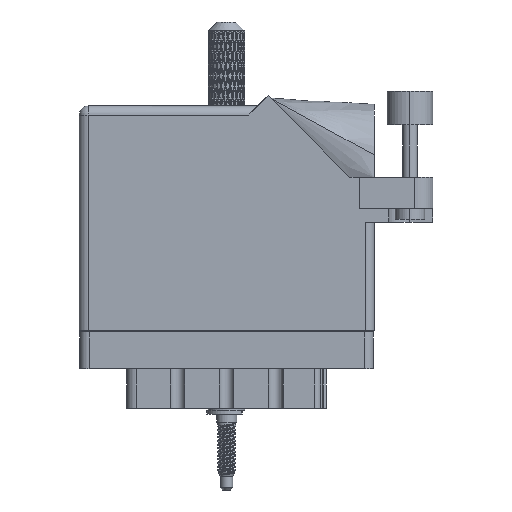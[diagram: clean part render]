
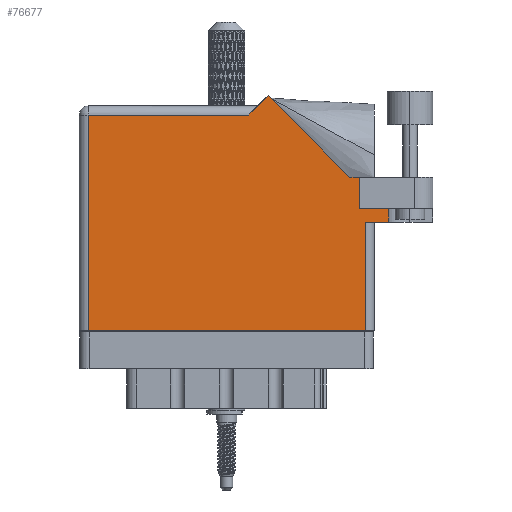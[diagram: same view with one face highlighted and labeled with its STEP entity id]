
A CAD part, front view. The second image highlights one B-rep face of the part: STEP entity #76677.
In plain terms, the highlighted face is planar.
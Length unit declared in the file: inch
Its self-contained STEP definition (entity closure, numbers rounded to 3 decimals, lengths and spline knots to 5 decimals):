
#57 = VECTOR ( 'NONE', #5268, 39.37008 ) ;
#938 = CARTESIAN_POINT ( 'NONE',  ( 0., 1.468, 0. ) ) ;
#1579 = LINE ( 'NONE', #55745, #51503 ) ;
#4344 = VECTOR ( 'NONE', #47164, 39.37008 ) ;
#4635 = DIRECTION ( 'NONE',  ( 1., 0., 0. ) ) ;
#5253 = VERTEX_POINT ( 'NONE', #78853 ) ;
#5268 = DIRECTION ( 'NONE',  ( -0.707, 0.707, 0. ) ) ;
#8035 = VERTEX_POINT ( 'NONE', #67696 ) ;
#8928 = VERTEX_POINT ( 'NONE', #51067 ) ;
#10046 = EDGE_CURVE ( 'NONE', #5253, #21552, #40392, .T. ) ;
#19671 = CARTESIAN_POINT ( 'NONE',  ( 1.948, 0.737, 0. ) ) ;
#21103 = DIRECTION ( 'NONE',  ( 1., 0., 0. ) ) ;
#21552 = VERTEX_POINT ( 'NONE', #83083 ) ;
#22017 = CARTESIAN_POINT ( 'NONE',  ( 1.84442, 1.044, 0. ) ) ;
#22342 = EDGE_CURVE ( 'NONE', #89152, #8035, #93505, .T. ) ;
#23425 = ORIENTED_EDGE ( 'NONE', *, *, #70591, .T. ) ;
#23950 = EDGE_CURVE ( 'NONE', #89152, #102067, #57091, .T. ) ;
#25335 = VERTEX_POINT ( 'NONE', #33425 ) ;
#25828 = VECTOR ( 'NONE', #78923, 39.37008 ) ;
#27591 = CARTESIAN_POINT ( 'NONE',  ( 0., 1.53, 0. ) ) ;
#28044 = VECTOR ( 'NONE', #87202, 39.37008 ) ;
#28593 = VECTOR ( 'NONE', #63120, 39.37008 ) ;
#28971 = CARTESIAN_POINT ( 'NONE',  ( 2.41, 1.044, 0. ) ) ;
#29723 = ORIENTED_EDGE ( 'NONE', *, *, #41947, .T. ) ;
#30612 = DIRECTION ( 'NONE',  ( 0., -1., 0. ) ) ;
#31033 = VECTOR ( 'NONE', #4635, 39.37008 ) ;
#32661 = EDGE_CURVE ( 'NONE', #8035, #25335, #1579, .T. ) ;
#32715 = ORIENTED_EDGE ( 'NONE', *, *, #77418, .T. ) ;
#33425 = CARTESIAN_POINT ( 'NONE',  ( 2.1115, 0.737, 0. ) ) ;
#34842 = VERTEX_POINT ( 'NONE', #71585 ) ;
#35898 = ORIENTED_EDGE ( 'NONE', *, *, #38329, .T. ) ;
#36081 = FACE_OUTER_BOUND ( 'NONE', #95447, .T. ) ;
#38329 = EDGE_CURVE ( 'NONE', #48681, #8928, #70773, .T. ) ;
#38809 = CARTESIAN_POINT ( 'NONE',  ( 1.948, 0.737, 0. ) ) ;
#40392 = LINE ( 'NONE', #938, #86519 ) ;
#41947 = EDGE_CURVE ( 'NONE', #82631, #25335, #71686, .T. ) ;
#42359 = LINE ( 'NONE', #66428, #62415 ) ;
#43043 = LINE ( 'NONE', #28971, #64299 ) ;
#43227 = CARTESIAN_POINT ( 'NONE',  ( 0.062, 0., 0. ) ) ;
#44780 = VERTEX_POINT ( 'NONE', #95991 ) ;
#47164 = DIRECTION ( 'NONE',  ( 0., 1., 0. ) ) ;
#47838 = ORIENTED_EDGE ( 'NONE', *, *, #75575, .T. ) ;
#48681 = VERTEX_POINT ( 'NONE', #43227 ) ;
#49773 = LINE ( 'NONE', #71113, #28593 ) ;
#50379 = CARTESIAN_POINT ( 'NONE',  ( 1.91, 1.044, 0. ) ) ;
#51067 = CARTESIAN_POINT ( 'NONE',  ( 1.948, 0., 0. ) ) ;
#51503 = VECTOR ( 'NONE', #30612, 39.37008 ) ;
#52007 = DIRECTION ( 'NONE',  ( 0., 0., -1. ) ) ;
#52464 = ORIENTED_EDGE ( 'NONE', *, *, #23950, .T. ) ;
#53269 = EDGE_CURVE ( 'NONE', #21552, #48681, #42359, .T. ) ;
#55745 = CARTESIAN_POINT ( 'NONE',  ( 2.1115, 1.16177, 0. ) ) ;
#56846 = CARTESIAN_POINT ( 'NONE',  ( 1.91, 0.831, 0. ) ) ;
#57091 = LINE ( 'NONE', #86573, #25828 ) ;
#57507 = LINE ( 'NONE', #22017, #57 ) ;
#57989 = LINE ( 'NONE', #38809, #4344 ) ;
#60066 = DIRECTION ( 'NONE',  ( -1., 0., 0. ) ) ;
#62415 = VECTOR ( 'NONE', #99236, 39.37008 ) ;
#62542 = ORIENTED_EDGE ( 'NONE', *, *, #10046, .T. ) ;
#62573 = AXIS2_PLACEMENT_3D ( 'NONE', #27591, #52007, #60066 ) ;
#63120 = DIRECTION ( 'NONE',  ( -0.707, -0.707, 0. ) ) ;
#64086 = DIRECTION ( 'NONE',  ( -1., 0., 0. ) ) ;
#64299 = VECTOR ( 'NONE', #85137, 39.37008 ) ;
#66428 = CARTESIAN_POINT ( 'NONE',  ( 0.062, 0., 0. ) ) ;
#67696 = CARTESIAN_POINT ( 'NONE',  ( 2.1115, 0.831, 0. ) ) ;
#69519 = CARTESIAN_POINT ( 'NONE',  ( 1.91, 0.831, 0. ) ) ;
#70591 = EDGE_CURVE ( 'NONE', #102067, #34842, #43043, .T. ) ;
#70773 = LINE ( 'NONE', #92269, #83317 ) ;
#71113 = CARTESIAN_POINT ( 'NONE',  ( 1.217, 1.53, 0. ) ) ;
#71585 = CARTESIAN_POINT ( 'NONE',  ( 1.84442, 1.044, 0. ) ) ;
#71686 = LINE ( 'NONE', #103572, #28044 ) ;
#71784 = EDGE_CURVE ( 'NONE', #8928, #82631, #57989, .T. ) ;
#72674 = ORIENTED_EDGE ( 'NONE', *, *, #32661, .F. ) ;
#75575 = EDGE_CURVE ( 'NONE', #34842, #44780, #57507, .T. ) ;
#76677 = ADVANCED_FACE ( 'NONE', ( #36081 ), #99842, .F. ) ;
#77418 = EDGE_CURVE ( 'NONE', #44780, #5253, #49773, .T. ) ;
#78853 = CARTESIAN_POINT ( 'NONE',  ( 1.155, 1.468, 0. ) ) ;
#78923 = DIRECTION ( 'NONE',  ( 0., 1., 0. ) ) ;
#79003 = ORIENTED_EDGE ( 'NONE', *, *, #71784, .T. ) ;
#82631 = VERTEX_POINT ( 'NONE', #19671 ) ;
#83083 = CARTESIAN_POINT ( 'NONE',  ( 0.062, 1.468, 0. ) ) ;
#83317 = VECTOR ( 'NONE', #21103, 39.37008 ) ;
#84419 = ORIENTED_EDGE ( 'NONE', *, *, #22342, .F. ) ;
#85137 = DIRECTION ( 'NONE',  ( -1., 0., 0. ) ) ;
#86519 = VECTOR ( 'NONE', #64086, 39.37008 ) ;
#86573 = CARTESIAN_POINT ( 'NONE',  ( 1.91, 0.831, 0. ) ) ;
#87050 = ORIENTED_EDGE ( 'NONE', *, *, #53269, .T. ) ;
#87202 = DIRECTION ( 'NONE',  ( 1., 0., 0. ) ) ;
#89152 = VERTEX_POINT ( 'NONE', #56846 ) ;
#92269 = CARTESIAN_POINT ( 'NONE',  ( 0., 0., 0. ) ) ;
#93505 = LINE ( 'NONE', #69519, #31033 ) ;
#95447 = EDGE_LOOP ( 'NONE', ( #35898, #79003, #29723, #72674, #84419, #52464, #23425, #47838, #32715, #62542, #87050 ) ) ;
#95991 = CARTESIAN_POINT ( 'NONE',  ( 1.28771, 1.60071, 0. ) ) ;
#99236 = DIRECTION ( 'NONE',  ( 0., -1., 0. ) ) ;
#99842 = PLANE ( 'NONE',  #62573 ) ;
#102067 = VERTEX_POINT ( 'NONE', #50379 ) ;
#103572 = CARTESIAN_POINT ( 'NONE',  ( 2.01, 0.737, 0. ) ) ;
